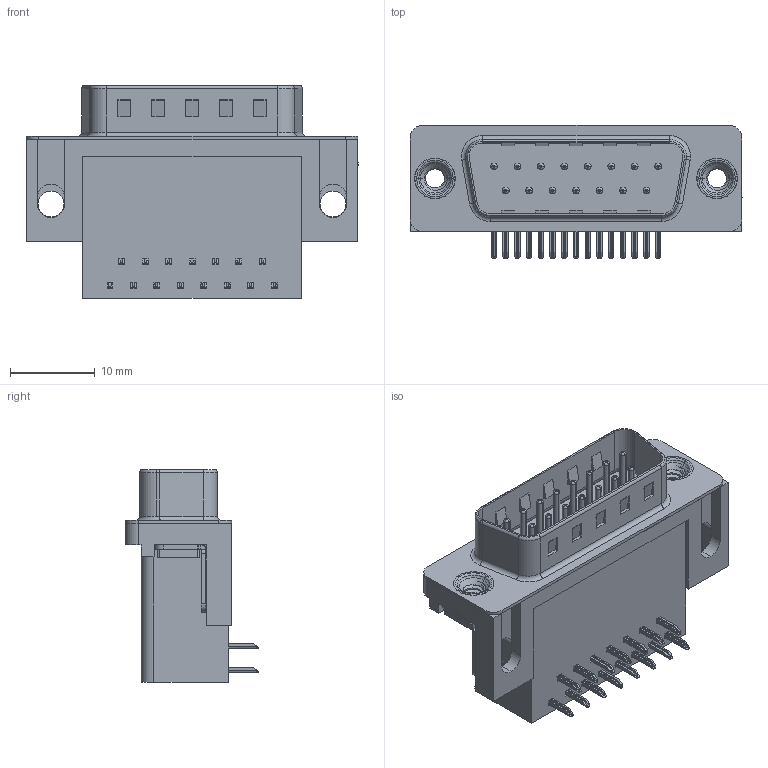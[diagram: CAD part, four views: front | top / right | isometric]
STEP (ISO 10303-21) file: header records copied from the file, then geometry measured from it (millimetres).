
FILE_DESCRIPTION (( 'STEP AP203' ), '1' );
FILE_NAME ('625-015-362-012.STEP', '2018-11-05T23:17:42', ( '' ), ( '' ), 'SwSTEP 2.0', 'SolidWorks 2016', '' );
FILE_SCHEMA (( 'CONFIG_CONTROL_DESIGN' ));
Length unit declared in the file: millimetre
Products named in the file (7): 625 Contact Top; 625 Thru Hole Board Mount; 625 4-40 Threaded Rivet; 625-015-362-012; 625 Housing_15 Socket; 625 Contact Bottom; 625 Shell_15 Socket
Assembly tree (21 placements, depth 2):
  625-015-362-012
    625 Housing_15 Socket
    625 Shell_15 Socket
    625 Contact Bottom  x7
    625 Contact Top  x8
    625 Thru Hole Board Mount  x2
    625 4-40 Threaded Rivet  x2
Bounding box: 39.22 x 15.73 x 25.16 mm (x, y, z)
Volume: 6241.6 mm3; surface area: 6411.8 mm2
Topology: 21 solids, 21 shells, 1479 faces, 3683 edges, 2283 vertices
Faces by surface type: plane 893, cylinder 447, torus 121, cone 12, bspline 6
Entity records: 19036 total; most frequent: CARTESIAN_POINT 4593, DIRECTION 2828, ORIENTED_EDGE 2718, EDGE_CURVE 1359, AXIS2_PLACEMENT_3D 952, LINE 924, VECTOR 924, VERTEX_POINT 867
